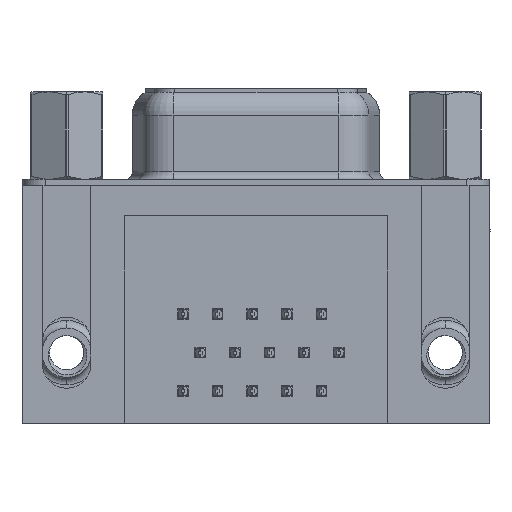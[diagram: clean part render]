
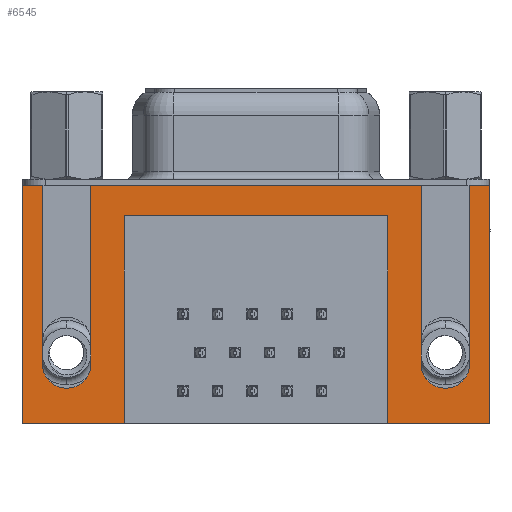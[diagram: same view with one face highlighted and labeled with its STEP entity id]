
A CAD part, front view. The second image highlights one B-rep face of the part: STEP entity #6545.
In plain terms, the highlighted planar face has unit normal (0, -1, 0).
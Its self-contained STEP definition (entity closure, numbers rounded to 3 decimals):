
#599 = CARTESIAN_POINT ( 'NONE',  ( 1.6, -6.275, 0. ) ) ;
#792 = DIRECTION ( 'NONE',  ( -1., 0., 0. ) ) ;
#901 = CARTESIAN_POINT ( 'NONE',  ( -2.91, -6.275, 0. ) ) ;
#1244 = VECTOR ( 'NONE', #1995, 1000. ) ;
#1289 = VECTOR ( 'NONE', #35628, 1000. ) ;
#1542 = AXIS2_PLACEMENT_3D ( 'NONE', #17114, #37230, #20581 ) ;
#1634 = VECTOR ( 'NONE', #29860, 1000. ) ;
#1660 = EDGE_CURVE ( 'NONE', #22542, #10215, #37515, .T. ) ;
#1741 = CARTESIAN_POINT ( 'NONE',  ( 27.9, -6.275, 0. ) ) ;
#1896 = CARTESIAN_POINT ( 'NONE',  ( 27.9, -6.275, -15.7 ) ) ;
#1995 = DIRECTION ( 'NONE',  ( 0., 0., -1. ) ) ;
#2294 = LINE ( 'NONE', #4145, #1244 ) ;
#3071 = CARTESIAN_POINT ( 'NONE',  ( -1.6, -6.275, -11.78 ) ) ;
#3279 = LINE ( 'NONE', #38261, #38027 ) ;
#3503 = VERTEX_POINT ( 'NONE', #599 ) ;
#3629 = LINE ( 'NONE', #15639, #13584 ) ;
#3990 = CARTESIAN_POINT ( 'NONE',  ( 27.9, -6.275, -15.7 ) ) ;
#4145 = CARTESIAN_POINT ( 'NONE',  ( 3.79, -6.275, -2. ) ) ;
#4708 = DIRECTION ( 'NONE',  ( 0., 0., 1. ) ) ;
#5341 = LINE ( 'NONE', #22733, #22352 ) ;
#5381 = VERTEX_POINT ( 'NONE', #30900 ) ;
#5467 = AXIS2_PLACEMENT_3D ( 'NONE', #23193, #33163, #12988 ) ;
#5721 = ORIENTED_EDGE ( 'NONE', *, *, #10662, .F. ) ;
#6125 = EDGE_CURVE ( 'NONE', #17824, #26243, #35940, .T. ) ;
#6341 = ORIENTED_EDGE ( 'NONE', *, *, #33711, .F. ) ;
#6545 = ADVANCED_FACE ( 'NONE', ( #31222 ), #9568, .T. ) ;
#6574 = CARTESIAN_POINT ( 'NONE',  ( 23.39, -6.275, -11.78 ) ) ;
#6707 = CARTESIAN_POINT ( 'NONE',  ( 26.59, -6.275, 0. ) ) ;
#7004 = ORIENTED_EDGE ( 'NONE', *, *, #34289, .F. ) ;
#7246 = ORIENTED_EDGE ( 'NONE', *, *, #32722, .F. ) ;
#7256 = VECTOR ( 'NONE', #24677, 1000. ) ;
#7792 = VECTOR ( 'NONE', #38750, 1000. ) ;
#8174 = CARTESIAN_POINT ( 'NONE',  ( 3.79, -6.275, -15.7 ) ) ;
#8315 = LINE ( 'NONE', #901, #7256 ) ;
#8734 = CARTESIAN_POINT ( 'NONE',  ( 21.2, -6.275, -15.7 ) ) ;
#8881 = EDGE_CURVE ( 'NONE', #5381, #8917, #30543, .T. ) ;
#8917 = VERTEX_POINT ( 'NONE', #37069 ) ;
#9284 = CARTESIAN_POINT ( 'NONE',  ( -2.91, -6.275, -15.7 ) ) ;
#9568 = PLANE ( 'NONE',  #5467 ) ;
#9789 = VERTEX_POINT ( 'NONE', #8734 ) ;
#10215 = VERTEX_POINT ( 'NONE', #31809 ) ;
#10462 = VERTEX_POINT ( 'NONE', #27153 ) ;
#10662 = EDGE_CURVE ( 'NONE', #3503, #34662, #8315, .T. ) ;
#11836 = CARTESIAN_POINT ( 'NONE',  ( 3.79, -6.275, -2. ) ) ;
#12519 = DIRECTION ( 'NONE',  ( 0., 0., 1. ) ) ;
#12988 = DIRECTION ( 'NONE',  ( 0., 0., -1. ) ) ;
#13052 = VECTOR ( 'NONE', #31088, 1000. ) ;
#13584 = VECTOR ( 'NONE', #26089, 1000. ) ;
#13902 = ORIENTED_EDGE ( 'NONE', *, *, #8881, .F. ) ;
#15139 = ORIENTED_EDGE ( 'NONE', *, *, #33216, .F. ) ;
#15179 = ORIENTED_EDGE ( 'NONE', *, *, #6125, .F. ) ;
#15639 = CARTESIAN_POINT ( 'NONE',  ( -1.6, -6.275, 0. ) ) ;
#15735 = LINE ( 'NONE', #18658, #7792 ) ;
#16409 = VECTOR ( 'NONE', #24847, 1000. ) ;
#16918 = LINE ( 'NONE', #29411, #23921 ) ;
#17114 = CARTESIAN_POINT ( 'NONE',  ( 0., -6.275, -11.78 ) ) ;
#17397 = CARTESIAN_POINT ( 'NONE',  ( 21.2, -6.275, -2. ) ) ;
#17505 = LINE ( 'NONE', #11836, #16409 ) ;
#17824 = VERTEX_POINT ( 'NONE', #33901 ) ;
#17864 = ORIENTED_EDGE ( 'NONE', *, *, #32917, .F. ) ;
#18658 = CARTESIAN_POINT ( 'NONE',  ( 1.6, -6.275, 0. ) ) ;
#19408 = DIRECTION ( 'NONE',  ( 0., 0., 1. ) ) ;
#20581 = DIRECTION ( 'NONE',  ( 1., 0., 0. ) ) ;
#20992 = DIRECTION ( 'NONE',  ( 0., -1., 0. ) ) ;
#21106 = LINE ( 'NONE', #3990, #13052 ) ;
#21189 = VECTOR ( 'NONE', #30331, 1000. ) ;
#21437 = VERTEX_POINT ( 'NONE', #27158 ) ;
#22119 = ORIENTED_EDGE ( 'NONE', *, *, #1660, .F. ) ;
#22352 = VECTOR ( 'NONE', #19408, 1000. ) ;
#22405 = CARTESIAN_POINT ( 'NONE',  ( -2.91, -6.275, 0. ) ) ;
#22542 = VERTEX_POINT ( 'NONE', #3071 ) ;
#22733 = CARTESIAN_POINT ( 'NONE',  ( 27.9, -6.275, -2.5 ) ) ;
#23193 = CARTESIAN_POINT ( 'NONE',  ( -2.91, -6.275, -2.5 ) ) ;
#23921 = VECTOR ( 'NONE', #12519, 1000. ) ;
#24677 = DIRECTION ( 'NONE',  ( 1., 0., 0. ) ) ;
#24847 = DIRECTION ( 'NONE',  ( -1., 0., 0. ) ) ;
#25123 = ORIENTED_EDGE ( 'NONE', *, *, #35003, .F. ) ;
#26089 = DIRECTION ( 'NONE',  ( 0., 0., -1. ) ) ;
#26229 = ORIENTED_EDGE ( 'NONE', *, *, #33844, .F. ) ;
#26243 = VERTEX_POINT ( 'NONE', #1741 ) ;
#26500 = VECTOR ( 'NONE', #42075, 1000. ) ;
#26973 = CIRCLE ( 'NONE', #35871, 1.6 ) ;
#27062 = CARTESIAN_POINT ( 'NONE',  ( -2.91, -6.275, 0. ) ) ;
#27153 = CARTESIAN_POINT ( 'NONE',  ( 26.59, -6.275, -11.78 ) ) ;
#27158 = CARTESIAN_POINT ( 'NONE',  ( 27.9, -6.275, -15.7 ) ) ;
#27519 = LINE ( 'NONE', #1896, #26500 ) ;
#28490 = LINE ( 'NONE', #33185, #1634 ) ;
#29048 = EDGE_CURVE ( 'NONE', #30970, #5381, #3279, .T. ) ;
#29269 = CARTESIAN_POINT ( 'NONE',  ( 23.39, -6.275, 0. ) ) ;
#29411 = CARTESIAN_POINT ( 'NONE',  ( 21.2, -6.275, -2. ) ) ;
#29860 = DIRECTION ( 'NONE',  ( 0., 0., -1. ) ) ;
#30161 = VERTEX_POINT ( 'NONE', #8174 ) ;
#30163 = VERTEX_POINT ( 'NONE', #31806 ) ;
#30331 = DIRECTION ( 'NONE',  ( 0., 0., 1. ) ) ;
#30338 = ORIENTED_EDGE ( 'NONE', *, *, #36246, .F. ) ;
#30352 = DIRECTION ( 'NONE',  ( 1., 0., 0. ) ) ;
#30399 = EDGE_LOOP ( 'NONE', ( #7246, #17864, #15139, #5721, #6341, #22119, #26229, #13902, #30749, #7004, #25123, #36425, #37095, #30338, #36198, #15179 ) ) ;
#30543 = LINE ( 'NONE', #27062, #38418 ) ;
#30749 = ORIENTED_EDGE ( 'NONE', *, *, #29048, .F. ) ;
#30900 = CARTESIAN_POINT ( 'NONE',  ( -2.91, -6.275, 0. ) ) ;
#30941 = EDGE_CURVE ( 'NONE', #21437, #26243, #5341, .T. ) ;
#30970 = VERTEX_POINT ( 'NONE', #9284 ) ;
#31088 = DIRECTION ( 'NONE',  ( -1., 0., 0. ) ) ;
#31222 = FACE_OUTER_BOUND ( 'NONE', #30399, .T. ) ;
#31806 = CARTESIAN_POINT ( 'NONE',  ( 3.79, -6.275, -2. ) ) ;
#31809 = CARTESIAN_POINT ( 'NONE',  ( 1.6, -6.275, -11.78 ) ) ;
#32722 = EDGE_CURVE ( 'NONE', #10462, #17824, #37913, .T. ) ;
#32917 = EDGE_CURVE ( 'NONE', #41364, #10462, #26973, .T. ) ;
#33163 = DIRECTION ( 'NONE',  ( 0., -1., 0. ) ) ;
#33185 = CARTESIAN_POINT ( 'NONE',  ( 23.39, -6.275, 0. ) ) ;
#33216 = EDGE_CURVE ( 'NONE', #34662, #41364, #28490, .T. ) ;
#33711 = EDGE_CURVE ( 'NONE', #10215, #3503, #15735, .T. ) ;
#33844 = EDGE_CURVE ( 'NONE', #8917, #22542, #3629, .T. ) ;
#33901 = CARTESIAN_POINT ( 'NONE',  ( 26.59, -6.275, 0. ) ) ;
#34289 = EDGE_CURVE ( 'NONE', #30161, #30970, #21106, .T. ) ;
#34662 = VERTEX_POINT ( 'NONE', #29269 ) ;
#35003 = EDGE_CURVE ( 'NONE', #30163, #30161, #2294, .T. ) ;
#35464 = EDGE_CURVE ( 'NONE', #38342, #30163, #17505, .T. ) ;
#35628 = DIRECTION ( 'NONE',  ( 1., 0., 0. ) ) ;
#35871 = AXIS2_PLACEMENT_3D ( 'NONE', #40973, #20992, #792 ) ;
#35940 = LINE ( 'NONE', #22405, #1289 ) ;
#35986 = EDGE_CURVE ( 'NONE', #9789, #38342, #16918, .T. ) ;
#36198 = ORIENTED_EDGE ( 'NONE', *, *, #30941, .T. ) ;
#36246 = EDGE_CURVE ( 'NONE', #21437, #9789, #27519, .T. ) ;
#36425 = ORIENTED_EDGE ( 'NONE', *, *, #35464, .F. ) ;
#37069 = CARTESIAN_POINT ( 'NONE',  ( -1.6, -6.275, 0. ) ) ;
#37095 = ORIENTED_EDGE ( 'NONE', *, *, #35986, .F. ) ;
#37230 = DIRECTION ( 'NONE',  ( 0., -1., 0. ) ) ;
#37515 = CIRCLE ( 'NONE', #1542, 1.6 ) ;
#37913 = LINE ( 'NONE', #6707, #21189 ) ;
#38027 = VECTOR ( 'NONE', #4708, 1000. ) ;
#38261 = CARTESIAN_POINT ( 'NONE',  ( -2.91, -6.275, -2.5 ) ) ;
#38342 = VERTEX_POINT ( 'NONE', #17397 ) ;
#38418 = VECTOR ( 'NONE', #30352, 1000. ) ;
#38750 = DIRECTION ( 'NONE',  ( 0., 0., 1. ) ) ;
#40973 = CARTESIAN_POINT ( 'NONE',  ( 24.99, -6.275, -11.78 ) ) ;
#41364 = VERTEX_POINT ( 'NONE', #6574 ) ;
#42075 = DIRECTION ( 'NONE',  ( -1., 0., 0. ) ) ;
